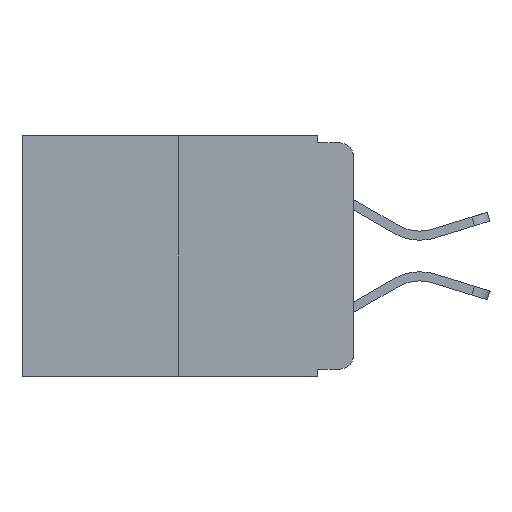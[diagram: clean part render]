
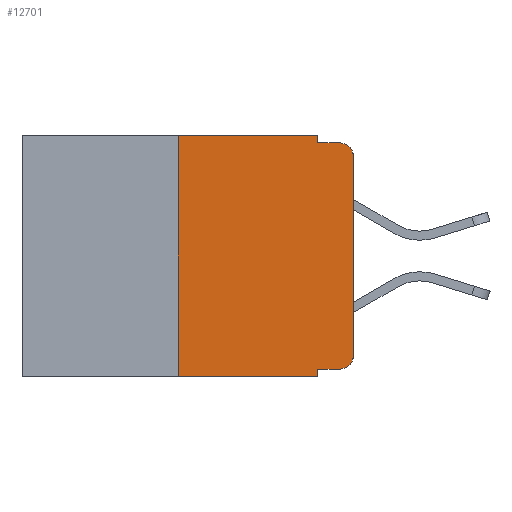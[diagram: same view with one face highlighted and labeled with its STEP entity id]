
A CAD part, left-side view. The second image highlights one B-rep face of the part: STEP entity #12701.
In plain terms, the highlighted planar face has unit normal (-1, 0, 0).
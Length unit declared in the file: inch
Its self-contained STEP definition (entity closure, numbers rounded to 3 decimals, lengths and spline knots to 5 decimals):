
#179 = CARTESIAN_POINT ( 'NONE',  ( 0., 0.051, -0.01 ) ) ;
#318 = CARTESIAN_POINT ( 'NONE',  ( 0., 0.473, -0.343 ) ) ;
#462 = LINE ( 'NONE', #12329, #24744 ) ;
#907 = VERTEX_POINT ( 'NONE', #10736 ) ;
#1001 = ORIENTED_EDGE ( 'NONE', *, *, #19734, .F. ) ;
#1535 = VERTEX_POINT ( 'NONE', #24931 ) ;
#1965 = AXIS2_PLACEMENT_3D ( 'NONE', #19356, #9681, #15304 ) ;
#2192 = EDGE_CURVE ( 'NONE', #16106, #21376, #13440, .T. ) ;
#2291 = VERTEX_POINT ( 'NONE', #6292 ) ;
#2584 = DIRECTION ( 'NONE',  ( 1., 0., 0. ) ) ;
#3946 = VECTOR ( 'NONE', #16339, 39.37008 ) ;
#4576 = FACE_OUTER_BOUND ( 'NONE', #9842, .T. ) ;
#4708 = AXIS2_PLACEMENT_3D ( 'NONE', #16406, #2584, #22173 ) ;
#5866 = DIRECTION ( 'NONE',  ( 0., 0., -1. ) ) ;
#5907 = ORIENTED_EDGE ( 'NONE', *, *, #2192, .T. ) ;
#6153 = AXIS2_PLACEMENT_3D ( 'NONE', #18411, #16320, #24334 ) ;
#6292 = CARTESIAN_POINT ( 'NONE',  ( 0., 0.051, -0.343 ) ) ;
#6493 = DIRECTION ( 'NONE',  ( 0., 0., 1. ) ) ;
#6573 = CIRCLE ( 'NONE', #1965, 0.02 ) ;
#7149 = VERTEX_POINT ( 'NONE', #21738 ) ;
#7177 = VERTEX_POINT ( 'NONE', #7589 ) ;
#7360 = VECTOR ( 'NONE', #18549, 39.37008 ) ;
#7589 = CARTESIAN_POINT ( 'NONE',  ( 0., 0.25, 0. ) ) ;
#7940 = EDGE_CURVE ( 'NONE', #16106, #2291, #16969, .T. ) ;
#8040 = CARTESIAN_POINT ( 'NONE',  ( 0., 0.02, -0.01 ) ) ;
#8687 = LINE ( 'NONE', #12530, #14959 ) ;
#8856 = EDGE_CURVE ( 'NONE', #1535, #20187, #13862, .T. ) ;
#8968 = DIRECTION ( 'NONE',  ( 0., -1., 0. ) ) ;
#9076 = EDGE_CURVE ( 'NONE', #13223, #11007, #19999, .T. ) ;
#9386 = DIRECTION ( 'NONE',  ( 0., -1., 0. ) ) ;
#9681 = DIRECTION ( 'NONE',  ( -1., 0., 0. ) ) ;
#9842 = EDGE_LOOP ( 'NONE', ( #15481, #21394, #15226, #17448, #1001, #14794, #23824, #10553, #5907, #22677 ) ) ;
#9982 = CARTESIAN_POINT ( 'NONE',  ( 0., 0.051, 0. ) ) ;
#10127 = EDGE_CURVE ( 'NONE', #907, #7177, #462, .T. ) ;
#10238 = VECTOR ( 'NONE', #9386, 39.37008 ) ;
#10325 = LINE ( 'NONE', #318, #3946 ) ;
#10553 = ORIENTED_EDGE ( 'NONE', *, *, #7940, .F. ) ;
#10736 = CARTESIAN_POINT ( 'NONE',  ( 0., 0.25, -0.343 ) ) ;
#11007 = VERTEX_POINT ( 'NONE', #8040 ) ;
#11721 = VECTOR ( 'NONE', #23440, 39.37008 ) ;
#11753 = VECTOR ( 'NONE', #5866, 39.37008 ) ;
#12329 = CARTESIAN_POINT ( 'NONE',  ( 0., 0.25, 0. ) ) ;
#12418 = DIRECTION ( 'NONE',  ( 0., -1., 0. ) ) ;
#12530 = CARTESIAN_POINT ( 'NONE',  ( 0., 0.473, 0. ) ) ;
#12701 = ADVANCED_FACE ( 'NONE', ( #4576 ), #16032, .F. ) ;
#12918 = CIRCLE ( 'NONE', #6153, 0.02 ) ;
#13223 = VERTEX_POINT ( 'NONE', #22631 ) ;
#13440 = LINE ( 'NONE', #15279, #10238 ) ;
#13862 = LINE ( 'NONE', #15827, #11721 ) ;
#14794 = ORIENTED_EDGE ( 'NONE', *, *, #10127, .F. ) ;
#14959 = VECTOR ( 'NONE', #8968, 39.37008 ) ;
#15226 = ORIENTED_EDGE ( 'NONE', *, *, #9076, .F. ) ;
#15279 = CARTESIAN_POINT ( 'NONE',  ( 0., 0.051, -0.333 ) ) ;
#15304 = DIRECTION ( 'NONE',  ( 0., 0., -1. ) ) ;
#15481 = ORIENTED_EDGE ( 'NONE', *, *, #8856, .T. ) ;
#15665 = EDGE_CURVE ( 'NONE', #907, #2291, #10325, .T. ) ;
#15827 = CARTESIAN_POINT ( 'NONE',  ( 0., 0., 0. ) ) ;
#16032 = PLANE ( 'NONE',  #4708 ) ;
#16106 = VERTEX_POINT ( 'NONE', #23132 ) ;
#16320 = DIRECTION ( 'NONE',  ( -1., 0., 0. ) ) ;
#16339 = DIRECTION ( 'NONE',  ( 0., -1., 0. ) ) ;
#16406 = CARTESIAN_POINT ( 'NONE',  ( 0., 0.473, 0. ) ) ;
#16969 = LINE ( 'NONE', #17098, #7360 ) ;
#17098 = CARTESIAN_POINT ( 'NONE',  ( 0., 0.051, 0. ) ) ;
#17150 = VECTOR ( 'NONE', #12418, 39.37008 ) ;
#17448 = ORIENTED_EDGE ( 'NONE', *, *, #22821, .F. ) ;
#18411 = CARTESIAN_POINT ( 'NONE',  ( 0., 0.02, -0.03 ) ) ;
#18549 = DIRECTION ( 'NONE',  ( 0., 0., -1. ) ) ;
#19356 = CARTESIAN_POINT ( 'NONE',  ( 0., 0.02, -0.313 ) ) ;
#19734 = EDGE_CURVE ( 'NONE', #7177, #7149, #8687, .T. ) ;
#19999 = LINE ( 'NONE', #179, #17150 ) ;
#20187 = VERTEX_POINT ( 'NONE', #20612 ) ;
#20612 = CARTESIAN_POINT ( 'NONE',  ( 0., 0., -0.03 ) ) ;
#20788 = EDGE_CURVE ( 'NONE', #21376, #1535, #6573, .T. ) ;
#20995 = EDGE_CURVE ( 'NONE', #20187, #11007, #12918, .T. ) ;
#21376 = VERTEX_POINT ( 'NONE', #22325 ) ;
#21394 = ORIENTED_EDGE ( 'NONE', *, *, #20995, .T. ) ;
#21738 = CARTESIAN_POINT ( 'NONE',  ( 0., 0.051, 0. ) ) ;
#21895 = LINE ( 'NONE', #9982, #11753 ) ;
#22173 = DIRECTION ( 'NONE',  ( 0., 0., -1. ) ) ;
#22325 = CARTESIAN_POINT ( 'NONE',  ( 0., 0.02, -0.333 ) ) ;
#22631 = CARTESIAN_POINT ( 'NONE',  ( 0., 0.051, -0.01 ) ) ;
#22677 = ORIENTED_EDGE ( 'NONE', *, *, #20788, .T. ) ;
#22821 = EDGE_CURVE ( 'NONE', #7149, #13223, #21895, .T. ) ;
#23132 = CARTESIAN_POINT ( 'NONE',  ( 0., 0.051, -0.333 ) ) ;
#23440 = DIRECTION ( 'NONE',  ( 0., 0., 1. ) ) ;
#23824 = ORIENTED_EDGE ( 'NONE', *, *, #15665, .T. ) ;
#24334 = DIRECTION ( 'NONE',  ( 0., 0., -1. ) ) ;
#24744 = VECTOR ( 'NONE', #6493, 39.37008 ) ;
#24931 = CARTESIAN_POINT ( 'NONE',  ( 0., 0., -0.313 ) ) ;
